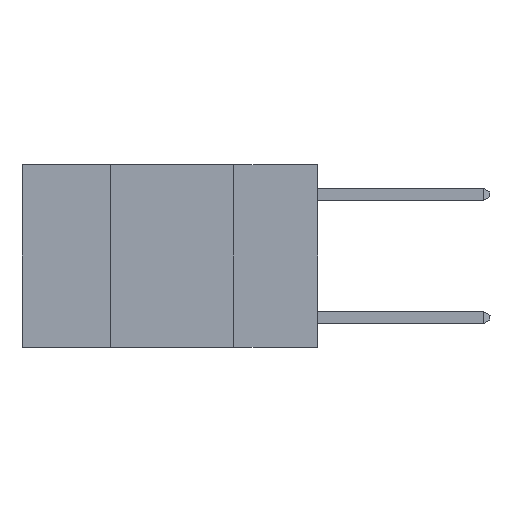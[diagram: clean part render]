
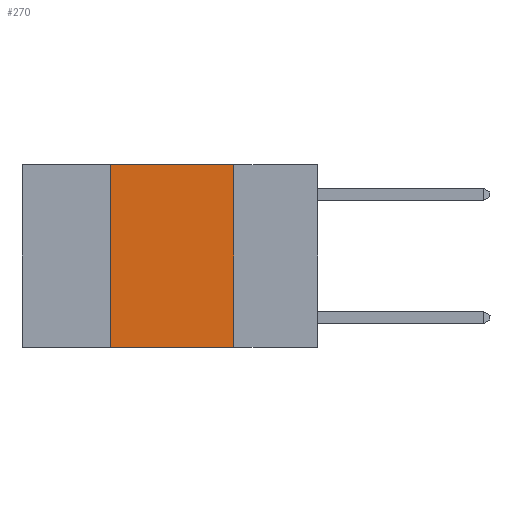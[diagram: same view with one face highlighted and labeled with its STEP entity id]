
A CAD part, left-side view. The second image highlights one B-rep face of the part: STEP entity #270.
In plain terms, the highlighted planar face has unit normal (-1, 0, 0).
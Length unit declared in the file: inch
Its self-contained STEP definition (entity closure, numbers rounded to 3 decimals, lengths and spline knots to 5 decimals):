
#270 = ADVANCED_FACE ( 'NONE', ( #6537 ), #523, .F. ) ;
#523 = PLANE ( 'NONE',  #12404 ) ;
#1666 = VERTEX_POINT ( 'NONE', #6053 ) ;
#1945 = VERTEX_POINT ( 'NONE', #3306 ) ;
#2294 = LINE ( 'NONE', #6767, #15589 ) ;
#2515 = ORIENTED_EDGE ( 'NONE', *, *, #14691, .F. ) ;
#2885 = LINE ( 'NONE', #10763, #3921 ) ;
#3021 = DIRECTION ( 'NONE',  ( 0., -1., 0. ) ) ;
#3306 = CARTESIAN_POINT ( 'NONE',  ( 0., 0.17, -0.37 ) ) ;
#3597 = ORIENTED_EDGE ( 'NONE', *, *, #8616, .F. ) ;
#3921 = VECTOR ( 'NONE', #3021, 39.37008 ) ;
#4278 = VECTOR ( 'NONE', #16546, 39.37008 ) ;
#4670 = CARTESIAN_POINT ( 'NONE',  ( 0., 0.17, 0. ) ) ;
#4672 = LINE ( 'NONE', #7582, #4278 ) ;
#5030 = ORIENTED_EDGE ( 'NONE', *, *, #13079, .T. ) ;
#5494 = DIRECTION ( 'NONE',  ( 0., -1., 0. ) ) ;
#6053 = CARTESIAN_POINT ( 'NONE',  ( 0., 0.17, 0. ) ) ;
#6537 = FACE_OUTER_BOUND ( 'NONE', #12860, .T. ) ;
#6767 = CARTESIAN_POINT ( 'NONE',  ( 0., 0.6, 0. ) ) ;
#6955 = DIRECTION ( 'NONE',  ( 1., 0., 0. ) ) ;
#7582 = CARTESIAN_POINT ( 'NONE',  ( 0., 0.42, 0. ) ) ;
#7913 = VECTOR ( 'NONE', #13604, 39.37008 ) ;
#8323 = LINE ( 'NONE', #4670, #7913 ) ;
#8616 = EDGE_CURVE ( 'NONE', #13657, #1666, #2294, .T. ) ;
#9557 = CARTESIAN_POINT ( 'NONE',  ( 0., 0.6, 0. ) ) ;
#10741 = DIRECTION ( 'NONE',  ( 0., 0., -1. ) ) ;
#10763 = CARTESIAN_POINT ( 'NONE',  ( 0., 0.6, -0.37 ) ) ;
#11256 = ORIENTED_EDGE ( 'NONE', *, *, #13267, .F. ) ;
#11413 = VERTEX_POINT ( 'NONE', #14743 ) ;
#12404 = AXIS2_PLACEMENT_3D ( 'NONE', #9557, #6955, #10741 ) ;
#12860 = EDGE_LOOP ( 'NONE', ( #11256, #3597, #2515, #5030 ) ) ;
#13079 = EDGE_CURVE ( 'NONE', #11413, #1945, #2885, .T. ) ;
#13267 = EDGE_CURVE ( 'NONE', #1666, #1945, #8323, .T. ) ;
#13604 = DIRECTION ( 'NONE',  ( 0., 0., -1. ) ) ;
#13657 = VERTEX_POINT ( 'NONE', #15768 ) ;
#14691 = EDGE_CURVE ( 'NONE', #11413, #13657, #4672, .T. ) ;
#14743 = CARTESIAN_POINT ( 'NONE',  ( 0., 0.42, -0.37 ) ) ;
#15589 = VECTOR ( 'NONE', #5494, 39.37008 ) ;
#15768 = CARTESIAN_POINT ( 'NONE',  ( 0., 0.42, 0. ) ) ;
#16546 = DIRECTION ( 'NONE',  ( 0., 0., 1. ) ) ;
